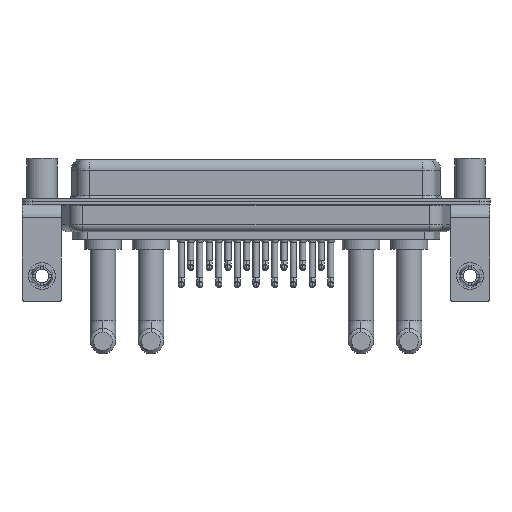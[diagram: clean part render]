
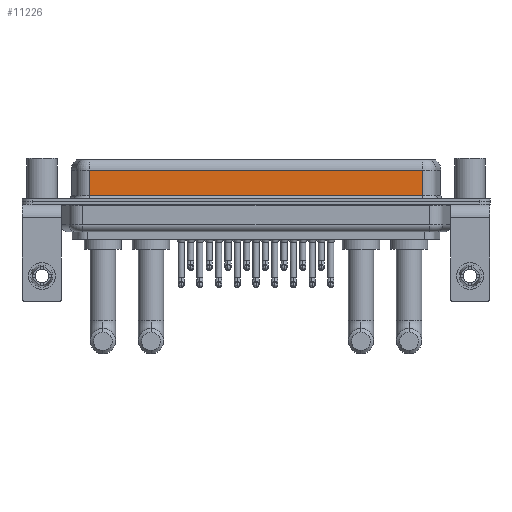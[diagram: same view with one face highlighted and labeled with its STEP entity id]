
A CAD part, front view. The second image highlights one B-rep face of the part: STEP entity #11226.
In plain terms, the highlighted planar face has unit normal (0, -1, 0).
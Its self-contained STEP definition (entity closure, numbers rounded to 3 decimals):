
#805 = EDGE_CURVE ( 'NONE', #2812, #16178, #7613, .T. ) ;
#1097 = VERTEX_POINT ( 'NONE', #1366 ) ;
#1314 = VERTEX_POINT ( 'NONE', #22281 ) ;
#1366 = CARTESIAN_POINT ( 'NONE',  ( 7.038, -3.95, 4.65 ) ) ;
#2812 = VERTEX_POINT ( 'NONE', #20558 ) ;
#3032 = ORIENTED_EDGE ( 'NONE', *, *, #5221, .T. ) ;
#3037 = CARTESIAN_POINT ( 'NONE',  ( 56.462, -3.95, 0.9 ) ) ;
#4484 = EDGE_CURVE ( 'NONE', #1097, #1314, #12107, .T. ) ;
#4968 = DIRECTION ( 'NONE',  ( 0., 0., 1. ) ) ;
#5221 = EDGE_CURVE ( 'NONE', #1314, #16178, #11395, .T. ) ;
#5300 = DIRECTION ( 'NONE',  ( 1., 0., 0. ) ) ;
#5851 = CARTESIAN_POINT ( 'NONE',  ( 56.462, -3.95, 4.65 ) ) ;
#6764 = ORIENTED_EDGE ( 'NONE', *, *, #805, .F. ) ;
#6962 = DIRECTION ( 'NONE',  ( 0., 1., 0. ) ) ;
#7352 = VECTOR ( 'NONE', #20067, 1000. ) ;
#7613 = LINE ( 'NONE', #18210, #7352 ) ;
#8777 = ORIENTED_EDGE ( 'NONE', *, *, #4484, .T. ) ;
#11195 = AXIS2_PLACEMENT_3D ( 'NONE', #20604, #6962, #4968 ) ;
#11226 = ADVANCED_FACE ( 'NONE', ( #16766 ), #14788, .F. ) ;
#11395 = LINE ( 'NONE', #19607, #22793 ) ;
#11820 = LINE ( 'NONE', #5851, #23358 ) ;
#12107 = LINE ( 'NONE', #22643, #18564 ) ;
#14706 = DIRECTION ( 'NONE',  ( 0., 0., -1. ) ) ;
#14788 = PLANE ( 'NONE',  #11195 ) ;
#16178 = VERTEX_POINT ( 'NONE', #3037 ) ;
#16766 = FACE_OUTER_BOUND ( 'NONE', #19874, .T. ) ;
#17332 = ORIENTED_EDGE ( 'NONE', *, *, #20678, .T. ) ;
#18036 = DIRECTION ( 'NONE',  ( -1., 0., 0. ) ) ;
#18210 = CARTESIAN_POINT ( 'NONE',  ( 56.462, -3.95, 6.4 ) ) ;
#18564 = VECTOR ( 'NONE', #14706, 1000. ) ;
#19607 = CARTESIAN_POINT ( 'NONE',  ( 56.462, -3.95, 0.9 ) ) ;
#19874 = EDGE_LOOP ( 'NONE', ( #6764, #17332, #8777, #3032 ) ) ;
#20067 = DIRECTION ( 'NONE',  ( 0., 0., -1. ) ) ;
#20558 = CARTESIAN_POINT ( 'NONE',  ( 56.462, -3.95, 4.65 ) ) ;
#20604 = CARTESIAN_POINT ( 'NONE',  ( 56.462, -3.95, 6.4 ) ) ;
#20678 = EDGE_CURVE ( 'NONE', #2812, #1097, #11820, .T. ) ;
#22281 = CARTESIAN_POINT ( 'NONE',  ( 7.038, -3.95, 0.9 ) ) ;
#22643 = CARTESIAN_POINT ( 'NONE',  ( 7.038, -3.95, 6.4 ) ) ;
#22793 = VECTOR ( 'NONE', #5300, 1000. ) ;
#23358 = VECTOR ( 'NONE', #18036, 1000. ) ;
